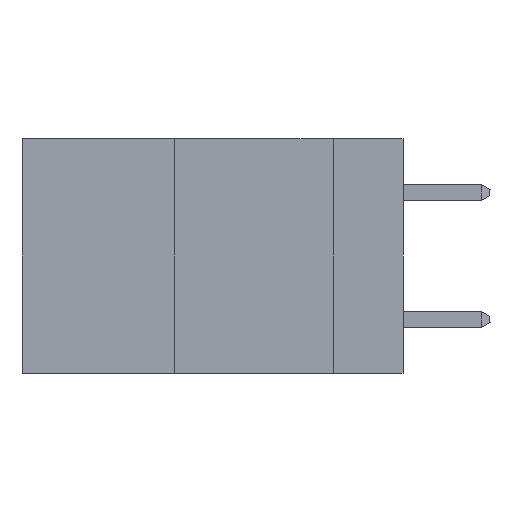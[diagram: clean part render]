
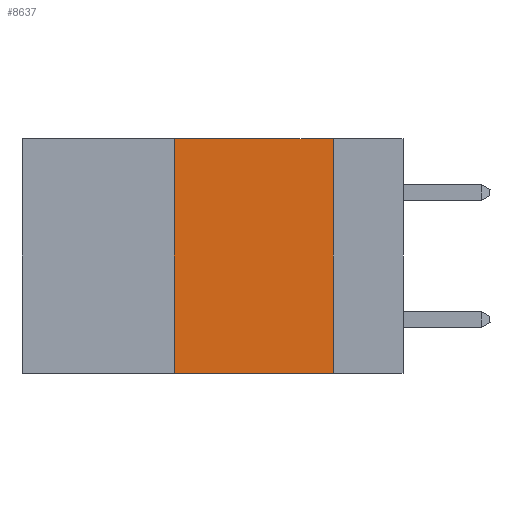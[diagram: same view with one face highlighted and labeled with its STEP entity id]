
A CAD part, left-side view. The second image highlights one B-rep face of the part: STEP entity #8637.
In plain terms, the highlighted planar face has unit normal (-1, 0, 0).
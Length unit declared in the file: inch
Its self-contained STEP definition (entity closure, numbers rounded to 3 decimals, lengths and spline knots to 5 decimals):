
#29 = CARTESIAN_POINT ( 'NONE',  ( 0., 0.6, -0.37 ) ) ;
#879 = ORIENTED_EDGE ( 'NONE', *, *, #14369, .F. ) ;
#943 = LINE ( 'NONE', #7925, #5775 ) ;
#1044 = CARTESIAN_POINT ( 'NONE',  ( 0., 0.6, 0. ) ) ;
#1106 = DIRECTION ( 'NONE',  ( 0., -1., 0. ) ) ;
#2054 = VECTOR ( 'NONE', #16156, 39.37008 ) ;
#2417 = AXIS2_PLACEMENT_3D ( 'NONE', #1044, #16643, #11974 ) ;
#2465 = EDGE_CURVE ( 'NONE', #17454, #3811, #943, .T. ) ;
#2917 = ORIENTED_EDGE ( 'NONE', *, *, #5296, .F. ) ;
#3662 = CARTESIAN_POINT ( 'NONE',  ( 0., 0.11, 0. ) ) ;
#3811 = VERTEX_POINT ( 'NONE', #10052 ) ;
#4172 = LINE ( 'NONE', #29, #17002 ) ;
#5219 = CARTESIAN_POINT ( 'NONE',  ( 0., 0.11, 0. ) ) ;
#5296 = EDGE_CURVE ( 'NONE', #19273, #11120, #10730, .T. ) ;
#5775 = VECTOR ( 'NONE', #17340, 39.37008 ) ;
#6343 = ORIENTED_EDGE ( 'NONE', *, *, #2465, .F. ) ;
#7455 = CARTESIAN_POINT ( 'NONE',  ( 0., 0.11, -0.37 ) ) ;
#7692 = FACE_OUTER_BOUND ( 'NONE', #18110, .T. ) ;
#7925 = CARTESIAN_POINT ( 'NONE',  ( 0., 0.36, 0. ) ) ;
#8637 = ADVANCED_FACE ( 'NONE', ( #7692 ), #16239, .F. ) ;
#10052 = CARTESIAN_POINT ( 'NONE',  ( 0., 0.36, 0. ) ) ;
#10558 = CARTESIAN_POINT ( 'NONE',  ( 0., 0.36, -0.37 ) ) ;
#10730 = LINE ( 'NONE', #3662, #2054 ) ;
#11120 = VERTEX_POINT ( 'NONE', #7455 ) ;
#11974 = DIRECTION ( 'NONE',  ( 0., 0., -1. ) ) ;
#13095 = ORIENTED_EDGE ( 'NONE', *, *, #18711, .T. ) ;
#14369 = EDGE_CURVE ( 'NONE', #3811, #19273, #16635, .T. ) ;
#16156 = DIRECTION ( 'NONE',  ( 0., 0., -1. ) ) ;
#16239 = PLANE ( 'NONE',  #2417 ) ;
#16635 = LINE ( 'NONE', #17799, #19564 ) ;
#16643 = DIRECTION ( 'NONE',  ( 1., 0., 0. ) ) ;
#16835 = DIRECTION ( 'NONE',  ( 0., -1., 0. ) ) ;
#17002 = VECTOR ( 'NONE', #16835, 39.37008 ) ;
#17340 = DIRECTION ( 'NONE',  ( 0., 0., 1. ) ) ;
#17454 = VERTEX_POINT ( 'NONE', #10558 ) ;
#17799 = CARTESIAN_POINT ( 'NONE',  ( 0., 0.6, 0. ) ) ;
#18110 = EDGE_LOOP ( 'NONE', ( #2917, #879, #6343, #13095 ) ) ;
#18711 = EDGE_CURVE ( 'NONE', #17454, #11120, #4172, .T. ) ;
#19273 = VERTEX_POINT ( 'NONE', #5219 ) ;
#19564 = VECTOR ( 'NONE', #1106, 39.37008 ) ;
